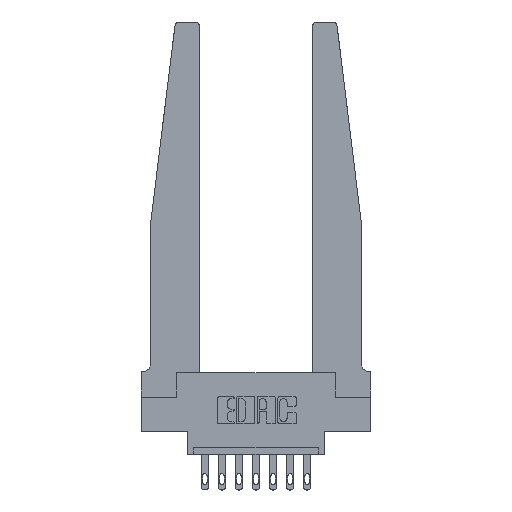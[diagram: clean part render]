
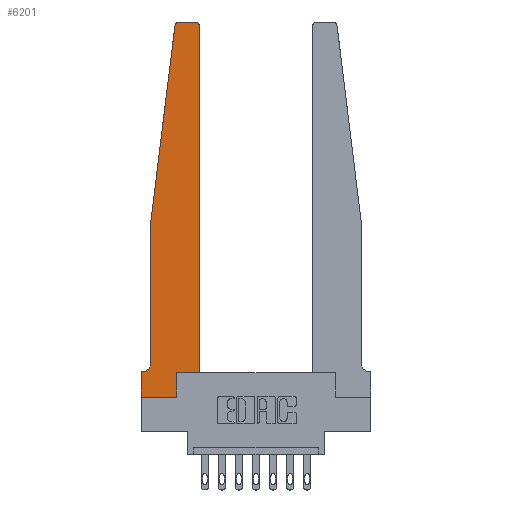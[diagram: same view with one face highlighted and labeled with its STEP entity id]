
A CAD part, top view. The second image highlights one B-rep face of the part: STEP entity #6201.
In plain terms, the highlighted planar face has unit normal (0, 0, 1).
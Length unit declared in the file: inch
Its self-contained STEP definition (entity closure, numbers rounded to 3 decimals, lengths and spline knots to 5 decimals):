
#2 = CARTESIAN_POINT ( 'NONE',  ( 0.065, 0.2375, 0.37 ) ) ;
#456 = ORIENTED_EDGE ( 'NONE', *, *, #5492, .T. ) ;
#645 = VERTEX_POINT ( 'NONE', #4215 ) ;
#699 = AXIS2_PLACEMENT_3D ( 'NONE', #1043, #7665, #12114 ) ;
#1043 = CARTESIAN_POINT ( 'NONE',  ( 0.395, 2.72, 0.37 ) ) ;
#1202 = EDGE_CURVE ( 'NONE', #645, #6872, #2527, .T. ) ;
#1267 = EDGE_CURVE ( 'NONE', #6307, #14189, #10337, .T. ) ;
#1304 = CARTESIAN_POINT ( 'NONE',  ( 0.2605, 0., 0.37 ) ) ;
#1322 = CARTESIAN_POINT ( 'NONE',  ( 0., 0., 0.37 ) ) ;
#1440 = DIRECTION ( 'NONE',  ( -1., 0., 0. ) ) ;
#1647 = VERTEX_POINT ( 'NONE', #2512 ) ;
#1830 = LINE ( 'NONE', #1901, #3063 ) ;
#1894 = AXIS2_PLACEMENT_3D ( 'NONE', #4721, #11578, #9402 ) ;
#1901 = CARTESIAN_POINT ( 'NONE',  ( 0.425, 0.18, 0.37 ) ) ;
#2108 = LINE ( 'NONE', #8766, #12854 ) ;
#2489 = EDGE_CURVE ( 'NONE', #3028, #4767, #2108, .T. ) ;
#2512 = CARTESIAN_POINT ( 'NONE',  ( 0.065, 1.25, 0.37 ) ) ;
#2527 = LINE ( 'NONE', #3459, #4772 ) ;
#2742 = CARTESIAN_POINT ( 'NONE',  ( 0.27653, 2.75, 0.37 ) ) ;
#2805 = CARTESIAN_POINT ( 'NONE',  ( 0.015, 0.1875, 0.37 ) ) ;
#2830 = VERTEX_POINT ( 'NONE', #7594 ) ;
#2914 = EDGE_CURVE ( 'NONE', #2830, #645, #5325, .T. ) ;
#2972 = DIRECTION ( 'NONE',  ( 1., 0., 0. ) ) ;
#3028 = VERTEX_POINT ( 'NONE', #1322 ) ;
#3063 = VECTOR ( 'NONE', #10657, 39.37008 ) ;
#3356 = ORIENTED_EDGE ( 'NONE', *, *, #1267, .T. ) ;
#3438 = VECTOR ( 'NONE', #12848, 39.37008 ) ;
#3459 = CARTESIAN_POINT ( 'NONE',  ( 0.25, 2.75, 0.37 ) ) ;
#4092 = ORIENTED_EDGE ( 'NONE', *, *, #10980, .T. ) ;
#4099 = EDGE_CURVE ( 'NONE', #1647, #7132, #5513, .T. ) ;
#4141 = DIRECTION ( 'NONE',  ( 0., 0., 1. ) ) ;
#4215 = CARTESIAN_POINT ( 'NONE',  ( 0.395, 2.75, 0.37 ) ) ;
#4403 = CARTESIAN_POINT ( 'NONE',  ( 0., 0.1875, 0.37 ) ) ;
#4434 = DIRECTION ( 'NONE',  ( 0., -1., 0. ) ) ;
#4551 = DIRECTION ( 'NONE',  ( 0., 0., 1. ) ) ;
#4721 = CARTESIAN_POINT ( 'NONE',  ( 0.015, 0.2375, 0.37 ) ) ;
#4743 = VECTOR ( 'NONE', #4434, 39.37008 ) ;
#4767 = VERTEX_POINT ( 'NONE', #1304 ) ;
#4772 = VECTOR ( 'NONE', #1440, 39.37008 ) ;
#4951 = LINE ( 'NONE', #10523, #9618 ) ;
#5238 = VECTOR ( 'NONE', #12636, 39.37008 ) ;
#5241 = CARTESIAN_POINT ( 'NONE',  ( 0.065, 0.1875, 0.37 ) ) ;
#5301 = CARTESIAN_POINT ( 'NONE',  ( 0.065, 1.25, 0.37 ) ) ;
#5325 = CIRCLE ( 'NONE', #699, 0.03 ) ;
#5492 = EDGE_CURVE ( 'NONE', #7132, #6008, #10915, .T. ) ;
#5503 = LINE ( 'NONE', #6727, #9044 ) ;
#5513 = LINE ( 'NONE', #5301, #4743 ) ;
#5521 = ORIENTED_EDGE ( 'NONE', *, *, #7796, .T. ) ;
#5617 = FACE_OUTER_BOUND ( 'NONE', #7679, .T. ) ;
#6008 = VERTEX_POINT ( 'NONE', #2805 ) ;
#6158 = LINE ( 'NONE', #13795, #5238 ) ;
#6201 = ADVANCED_FACE ( 'NONE', ( #5617 ), #10985, .T. ) ;
#6212 = DIRECTION ( 'NONE',  ( 1., 0., 0. ) ) ;
#6307 = VERTEX_POINT ( 'NONE', #11768 ) ;
#6363 = VECTOR ( 'NONE', #13536, 39.37008 ) ;
#6727 = CARTESIAN_POINT ( 'NONE',  ( 0.2605, 0.18, 0.37 ) ) ;
#6872 = VERTEX_POINT ( 'NONE', #2742 ) ;
#6891 = ORIENTED_EDGE ( 'NONE', *, *, #13035, .T. ) ;
#7091 = ORIENTED_EDGE ( 'NONE', *, *, #1202, .T. ) ;
#7132 = VERTEX_POINT ( 'NONE', #2 ) ;
#7370 = CARTESIAN_POINT ( 'NONE',  ( 0.27653, 2.72, 0.37 ) ) ;
#7594 = CARTESIAN_POINT ( 'NONE',  ( 0.425, 2.72, 0.37 ) ) ;
#7648 = AXIS2_PLACEMENT_3D ( 'NONE', #7370, #4141, #6212 ) ;
#7665 = DIRECTION ( 'NONE',  ( 0., 0., 1. ) ) ;
#7679 = EDGE_LOOP ( 'NONE', ( #7091, #6891, #4092, #8712, #456, #5521, #8122, #8985, #9936, #3356, #10070, #8218 ) ) ;
#7764 = CARTESIAN_POINT ( 'NONE',  ( 0.425, 0.18, 0.37 ) ) ;
#7796 = EDGE_CURVE ( 'NONE', #6008, #10166, #11903, .T. ) ;
#8102 = CARTESIAN_POINT ( 'NONE',  ( 0., 0.1875, 0.37 ) ) ;
#8122 = ORIENTED_EDGE ( 'NONE', *, *, #11101, .T. ) ;
#8149 = CARTESIAN_POINT ( 'NONE',  ( 0.425, 0.18, 0.37 ) ) ;
#8218 = ORIENTED_EDGE ( 'NONE', *, *, #2914, .T. ) ;
#8712 = ORIENTED_EDGE ( 'NONE', *, *, #4099, .T. ) ;
#8766 = CARTESIAN_POINT ( 'NONE',  ( 0., 0., 0.37 ) ) ;
#8942 = DIRECTION ( 'NONE',  ( 1., 0., 0. ) ) ;
#8985 = ORIENTED_EDGE ( 'NONE', *, *, #2489, .T. ) ;
#9044 = VECTOR ( 'NONE', #9918, 39.37008 ) ;
#9402 = DIRECTION ( 'NONE',  ( -1., 0., 0. ) ) ;
#9618 = VECTOR ( 'NONE', #11675, 39.37008 ) ;
#9915 = EDGE_CURVE ( 'NONE', #14189, #2830, #1830, .T. ) ;
#9918 = DIRECTION ( 'NONE',  ( 0., 1., 0. ) ) ;
#9936 = ORIENTED_EDGE ( 'NONE', *, *, #13281, .T. ) ;
#10070 = ORIENTED_EDGE ( 'NONE', *, *, #9915, .T. ) ;
#10166 = VERTEX_POINT ( 'NONE', #8102 ) ;
#10337 = LINE ( 'NONE', #8149, #6363 ) ;
#10523 = CARTESIAN_POINT ( 'NONE',  ( 0., 0., 0.37 ) ) ;
#10657 = DIRECTION ( 'NONE',  ( 0., 1., 0. ) ) ;
#10915 = CIRCLE ( 'NONE', #1894, 0.05 ) ;
#10980 = EDGE_CURVE ( 'NONE', #13290, #1647, #6158, .T. ) ;
#10985 = PLANE ( 'NONE',  #13235 ) ;
#11101 = EDGE_CURVE ( 'NONE', #10166, #3028, #4951, .T. ) ;
#11578 = DIRECTION ( 'NONE',  ( 0., 0., -1. ) ) ;
#11675 = DIRECTION ( 'NONE',  ( 0., -1., 0. ) ) ;
#11768 = CARTESIAN_POINT ( 'NONE',  ( 0.2605, 0.18, 0.37 ) ) ;
#11903 = LINE ( 'NONE', #5241, #3438 ) ;
#11958 = CARTESIAN_POINT ( 'NONE',  ( 0.24675, 2.72367, 0.37 ) ) ;
#12114 = DIRECTION ( 'NONE',  ( 1., 0., 0. ) ) ;
#12636 = DIRECTION ( 'NONE',  ( -0.122, -0.992, 0. ) ) ;
#12848 = DIRECTION ( 'NONE',  ( -1., 0., 0. ) ) ;
#12854 = VECTOR ( 'NONE', #2972, 39.37008 ) ;
#13035 = EDGE_CURVE ( 'NONE', #6872, #13290, #13194, .T. ) ;
#13194 = CIRCLE ( 'NONE', #7648, 0.03 ) ;
#13235 = AXIS2_PLACEMENT_3D ( 'NONE', #4403, #4551, #8942 ) ;
#13281 = EDGE_CURVE ( 'NONE', #4767, #6307, #5503, .T. ) ;
#13290 = VERTEX_POINT ( 'NONE', #11958 ) ;
#13536 = DIRECTION ( 'NONE',  ( 1., 0., 0. ) ) ;
#13795 = CARTESIAN_POINT ( 'NONE',  ( 0.065, 1.25, 0.37 ) ) ;
#14189 = VERTEX_POINT ( 'NONE', #7764 ) ;
